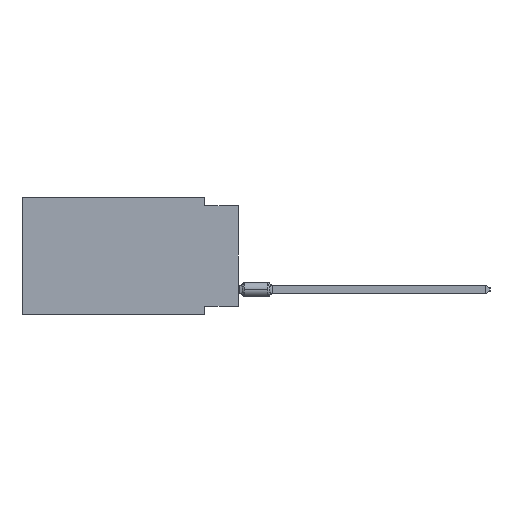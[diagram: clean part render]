
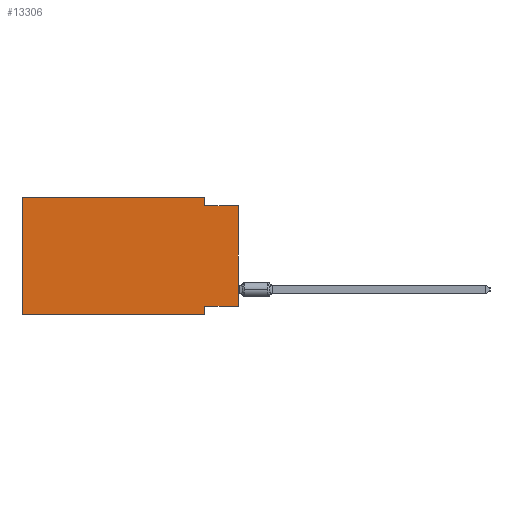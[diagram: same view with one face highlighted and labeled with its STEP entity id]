
A CAD part, left-side view. The second image highlights one B-rep face of the part: STEP entity #13306.
In plain terms, the highlighted planar face has unit normal (-1, 0, 0).
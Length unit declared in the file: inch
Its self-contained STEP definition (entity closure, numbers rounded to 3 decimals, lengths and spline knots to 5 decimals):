
#3056 = DIRECTION ( 'NONE',  ( 0., -1., 0. ) ) ;
#4973 = FACE_OUTER_BOUND ( 'NONE', #21304, .T. ) ;
#6489 = LINE ( 'NONE', #90585, #9955 ) ;
#8464 = CARTESIAN_POINT ( 'NONE',  ( 0., 0.645, 0. ) ) ;
#9955 = VECTOR ( 'NONE', #16338, 39.37008 ) ;
#10803 = VERTEX_POINT ( 'NONE', #81272 ) ;
#11292 = LINE ( 'NONE', #78382, #23929 ) ;
#11354 = EDGE_CURVE ( 'NONE', #58048, #33125, #16726, .T. ) ;
#13306 = ADVANCED_FACE ( 'NONE', ( #4973 ), #105053, .F. ) ;
#16338 = DIRECTION ( 'NONE',  ( 0., 0., 1. ) ) ;
#16726 = LINE ( 'NONE', #8464, #52444 ) ;
#17042 = VERTEX_POINT ( 'NONE', #97404 ) ;
#21304 = EDGE_LOOP ( 'NONE', ( #60494, #55975, #87155, #38796, #68813, #43087, #34327, #25175 ) ) ;
#22960 = CARTESIAN_POINT ( 'NONE',  ( 0., 0.1, -0.35 ) ) ;
#23929 = VECTOR ( 'NONE', #3056, 39.37008 ) ;
#25175 = ORIENTED_EDGE ( 'NONE', *, *, #105130, .F. ) ;
#27392 = VECTOR ( 'NONE', #56614, 39.37008 ) ;
#31010 = VERTEX_POINT ( 'NONE', #49640 ) ;
#31353 = VERTEX_POINT ( 'NONE', #79273 ) ;
#33125 = VERTEX_POINT ( 'NONE', #75236 ) ;
#34327 = ORIENTED_EDGE ( 'NONE', *, *, #56852, .F. ) ;
#38796 = ORIENTED_EDGE ( 'NONE', *, *, #11354, .F. ) ;
#39946 = DIRECTION ( 'NONE',  ( 0., 0., -1. ) ) ;
#40296 = LINE ( 'NONE', #73829, #78685 ) ;
#41479 = DIRECTION ( 'NONE',  ( 0., -1., 0. ) ) ;
#43087 = ORIENTED_EDGE ( 'NONE', *, *, #103523, .T. ) ;
#43592 = EDGE_CURVE ( 'NONE', #71648, #56375, #6489, .T. ) ;
#45643 = VECTOR ( 'NONE', #39946, 39.37008 ) ;
#49085 = VECTOR ( 'NONE', #56913, 39.37008 ) ;
#49640 = CARTESIAN_POINT ( 'NONE',  ( 0., 0.645, -0.35 ) ) ;
#52225 = EDGE_CURVE ( 'NONE', #31010, #58048, #40296, .T. ) ;
#52444 = VECTOR ( 'NONE', #41479, 39.37008 ) ;
#55544 = DIRECTION ( 'NONE',  ( 1., 0., 0. ) ) ;
#55975 = ORIENTED_EDGE ( 'NONE', *, *, #64668, .F. ) ;
#56375 = VERTEX_POINT ( 'NONE', #106119 ) ;
#56614 = DIRECTION ( 'NONE',  ( 0., 1., 0. ) ) ;
#56852 = EDGE_CURVE ( 'NONE', #17042, #31353, #66328, .T. ) ;
#56913 = DIRECTION ( 'NONE',  ( 0., -1., 0. ) ) ;
#57789 = CARTESIAN_POINT ( 'NONE',  ( 0., 0., -0.325 ) ) ;
#58048 = VERTEX_POINT ( 'NONE', #108289 ) ;
#60494 = ORIENTED_EDGE ( 'NONE', *, *, #43592, .T. ) ;
#61783 = VECTOR ( 'NONE', #107615, 39.37008 ) ;
#64313 = LINE ( 'NONE', #97307, #27392 ) ;
#64668 = EDGE_CURVE ( 'NONE', #10803, #56375, #11292, .T. ) ;
#66328 = LINE ( 'NONE', #22960, #61783 ) ;
#68813 = ORIENTED_EDGE ( 'NONE', *, *, #52225, .F. ) ;
#71648 = VERTEX_POINT ( 'NONE', #57789 ) ;
#73829 = CARTESIAN_POINT ( 'NONE',  ( 0., 0.645, 0. ) ) ;
#75236 = CARTESIAN_POINT ( 'NONE',  ( 0., 0.1, 0. ) ) ;
#78382 = CARTESIAN_POINT ( 'NONE',  ( 0., 0., -0.025 ) ) ;
#78685 = VECTOR ( 'NONE', #96380, 39.37008 ) ;
#79273 = CARTESIAN_POINT ( 'NONE',  ( 0., 0.1, -0.35 ) ) ;
#80869 = CARTESIAN_POINT ( 'NONE',  ( 0., 0.645, 0. ) ) ;
#81272 = CARTESIAN_POINT ( 'NONE',  ( 0., 0.1, -0.025 ) ) ;
#82811 = CARTESIAN_POINT ( 'NONE',  ( 0., 0.1, 0. ) ) ;
#84426 = EDGE_CURVE ( 'NONE', #33125, #10803, #91050, .T. ) ;
#87155 = ORIENTED_EDGE ( 'NONE', *, *, #84426, .F. ) ;
#89654 = DIRECTION ( 'NONE',  ( 0., 0., -1. ) ) ;
#90585 = CARTESIAN_POINT ( 'NONE',  ( 0., 0., 0. ) ) ;
#91050 = LINE ( 'NONE', #82811, #45643 ) ;
#91383 = AXIS2_PLACEMENT_3D ( 'NONE', #80869, #55544, #89654 ) ;
#96380 = DIRECTION ( 'NONE',  ( 0., 0., 1. ) ) ;
#97307 = CARTESIAN_POINT ( 'NONE',  ( 0., 0., -0.325 ) ) ;
#97404 = CARTESIAN_POINT ( 'NONE',  ( 0., 0.1, -0.325 ) ) ;
#98162 = CARTESIAN_POINT ( 'NONE',  ( 0., 0.645, -0.35 ) ) ;
#103523 = EDGE_CURVE ( 'NONE', #31010, #31353, #108025, .T. ) ;
#105053 = PLANE ( 'NONE',  #91383 ) ;
#105130 = EDGE_CURVE ( 'NONE', #71648, #17042, #64313, .T. ) ;
#106119 = CARTESIAN_POINT ( 'NONE',  ( 0., 0., -0.025 ) ) ;
#107615 = DIRECTION ( 'NONE',  ( 0., 0., -1. ) ) ;
#108025 = LINE ( 'NONE', #98162, #49085 ) ;
#108289 = CARTESIAN_POINT ( 'NONE',  ( 0., 0.645, 0. ) ) ;
